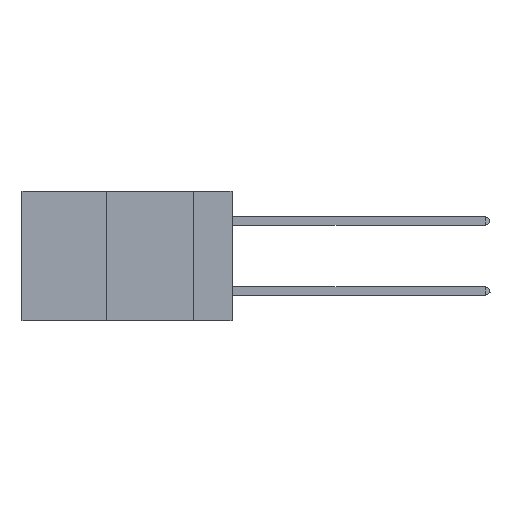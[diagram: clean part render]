
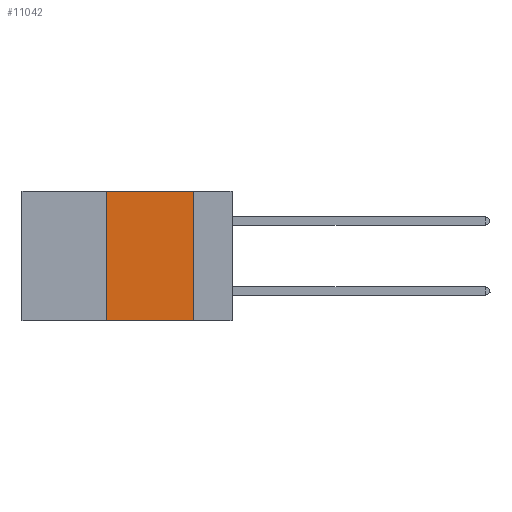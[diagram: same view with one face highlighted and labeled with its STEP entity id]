
A CAD part, left-side view. The second image highlights one B-rep face of the part: STEP entity #11042.
In plain terms, the highlighted planar face has unit normal (-1, 0, 0).
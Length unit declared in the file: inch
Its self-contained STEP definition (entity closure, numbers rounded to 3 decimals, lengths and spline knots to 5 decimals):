
#332 = VECTOR ( 'NONE', #8100, 39.37008 ) ;
#1240 = LINE ( 'NONE', #1969, #10567 ) ;
#1969 = CARTESIAN_POINT ( 'NONE',  ( 0., 0.36, 0. ) ) ;
#2083 = EDGE_CURVE ( 'NONE', #9373, #8348, #1240, .T. ) ;
#2502 = AXIS2_PLACEMENT_3D ( 'NONE', #6913, #11552, #4891 ) ;
#2794 = EDGE_CURVE ( 'NONE', #9373, #3221, #10542, .T. ) ;
#2968 = ORIENTED_EDGE ( 'NONE', *, *, #2083, .F. ) ;
#3221 = VERTEX_POINT ( 'NONE', #10102 ) ;
#4891 = DIRECTION ( 'NONE',  ( 0., 0., -1. ) ) ;
#5423 = FACE_OUTER_BOUND ( 'NONE', #9388, .T. ) ;
#5561 = CARTESIAN_POINT ( 'NONE',  ( 0., 0.6, 0. ) ) ;
#5685 = ORIENTED_EDGE ( 'NONE', *, *, #10469, .F. ) ;
#5961 = DIRECTION ( 'NONE',  ( 0., 0., -1. ) ) ;
#6723 = ORIENTED_EDGE ( 'NONE', *, *, #10879, .F. ) ;
#6913 = CARTESIAN_POINT ( 'NONE',  ( 0., 0.6, 0. ) ) ;
#7140 = CARTESIAN_POINT ( 'NONE',  ( 0., 0.6, -0.37 ) ) ;
#7522 = VECTOR ( 'NONE', #11318, 39.37008 ) ;
#7877 = VECTOR ( 'NONE', #5961, 39.37008 ) ;
#8083 = VERTEX_POINT ( 'NONE', #10655 ) ;
#8100 = DIRECTION ( 'NONE',  ( 0., -1., 0. ) ) ;
#8294 = ORIENTED_EDGE ( 'NONE', *, *, #2794, .T. ) ;
#8348 = VERTEX_POINT ( 'NONE', #9428 ) ;
#8633 = LINE ( 'NONE', #11598, #7877 ) ;
#9373 = VERTEX_POINT ( 'NONE', #9805 ) ;
#9388 = EDGE_LOOP ( 'NONE', ( #5685, #6723, #2968, #8294 ) ) ;
#9428 = CARTESIAN_POINT ( 'NONE',  ( 0., 0.36, 0. ) ) ;
#9805 = CARTESIAN_POINT ( 'NONE',  ( 0., 0.36, -0.37 ) ) ;
#10028 = LINE ( 'NONE', #5561, #7522 ) ;
#10102 = CARTESIAN_POINT ( 'NONE',  ( 0., 0.11, -0.37 ) ) ;
#10469 = EDGE_CURVE ( 'NONE', #8083, #3221, #8633, .T. ) ;
#10515 = PLANE ( 'NONE',  #2502 ) ;
#10542 = LINE ( 'NONE', #7140, #332 ) ;
#10567 = VECTOR ( 'NONE', #11520, 39.37008 ) ;
#10655 = CARTESIAN_POINT ( 'NONE',  ( 0., 0.11, 0. ) ) ;
#10879 = EDGE_CURVE ( 'NONE', #8348, #8083, #10028, .T. ) ;
#11042 = ADVANCED_FACE ( 'NONE', ( #5423 ), #10515, .F. ) ;
#11318 = DIRECTION ( 'NONE',  ( 0., -1., 0. ) ) ;
#11520 = DIRECTION ( 'NONE',  ( 0., 0., 1. ) ) ;
#11552 = DIRECTION ( 'NONE',  ( 1., 0., 0. ) ) ;
#11598 = CARTESIAN_POINT ( 'NONE',  ( 0., 0.11, 0. ) ) ;
